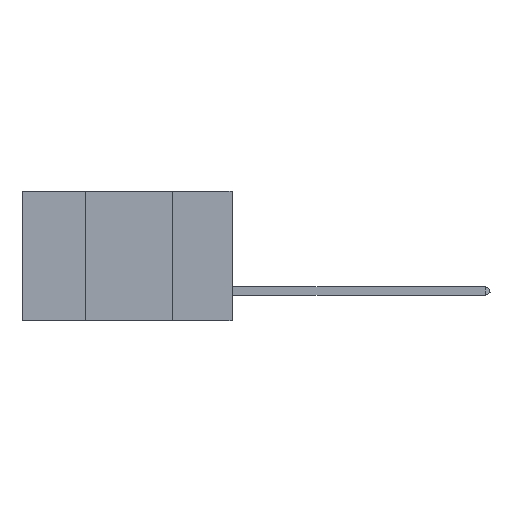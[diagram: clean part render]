
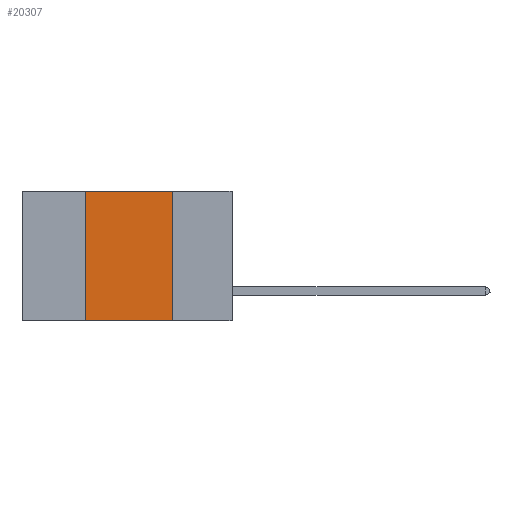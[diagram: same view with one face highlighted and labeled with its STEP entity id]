
A CAD part, left-side view. The second image highlights one B-rep face of the part: STEP entity #20307.
In plain terms, the highlighted planar face has unit normal (-1, 0, 0).
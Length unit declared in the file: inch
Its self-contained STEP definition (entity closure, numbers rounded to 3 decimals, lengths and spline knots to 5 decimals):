
#463 = DIRECTION ( 'NONE',  ( 1., 0., 0. ) ) ;
#1718 = LINE ( 'NONE', #19362, #26135 ) ;
#1923 = CARTESIAN_POINT ( 'NONE',  ( 0., 0.6, -0.37 ) ) ;
#3035 = PLANE ( 'NONE',  #10450 ) ;
#4197 = CARTESIAN_POINT ( 'NONE',  ( 0., 0.17, -0.37 ) ) ;
#4352 = EDGE_CURVE ( 'NONE', #13098, #8558, #22935, .T. ) ;
#4533 = CARTESIAN_POINT ( 'NONE',  ( 0., 0.42, 0. ) ) ;
#4908 = LINE ( 'NONE', #24232, #18678 ) ;
#5317 = DIRECTION ( 'NONE',  ( 0., 0., -1. ) ) ;
#5902 = CARTESIAN_POINT ( 'NONE',  ( 0., 0.42, -0.37 ) ) ;
#6944 = VERTEX_POINT ( 'NONE', #4197 ) ;
#8126 = LINE ( 'NONE', #1923, #8457 ) ;
#8192 = EDGE_CURVE ( 'NONE', #13098, #6944, #8126, .T. ) ;
#8457 = VECTOR ( 'NONE', #8858, 39.37008 ) ;
#8558 = VERTEX_POINT ( 'NONE', #12243 ) ;
#8695 = EDGE_CURVE ( 'NONE', #8558, #15946, #4908, .T. ) ;
#8858 = DIRECTION ( 'NONE',  ( 0., -1., 0. ) ) ;
#9001 = FACE_OUTER_BOUND ( 'NONE', #20872, .T. ) ;
#10450 = AXIS2_PLACEMENT_3D ( 'NONE', #14301, #463, #5317 ) ;
#12243 = CARTESIAN_POINT ( 'NONE',  ( 0., 0.42, 0. ) ) ;
#13098 = VERTEX_POINT ( 'NONE', #5902 ) ;
#14301 = CARTESIAN_POINT ( 'NONE',  ( 0., 0.6, 0. ) ) ;
#15802 = DIRECTION ( 'NONE',  ( 0., 0., 1. ) ) ;
#15946 = VERTEX_POINT ( 'NONE', #19304 ) ;
#16084 = ORIENTED_EDGE ( 'NONE', *, *, #4352, .F. ) ;
#18678 = VECTOR ( 'NONE', #19539, 39.37008 ) ;
#19304 = CARTESIAN_POINT ( 'NONE',  ( 0., 0.17, 0. ) ) ;
#19362 = CARTESIAN_POINT ( 'NONE',  ( 0., 0.17, 0. ) ) ;
#19539 = DIRECTION ( 'NONE',  ( 0., -1., 0. ) ) ;
#20307 = ADVANCED_FACE ( 'NONE', ( #9001 ), #3035, .F. ) ;
#20872 = EDGE_LOOP ( 'NONE', ( #21194, #29105, #16084, #26406 ) ) ;
#21194 = ORIENTED_EDGE ( 'NONE', *, *, #23361, .F. ) ;
#22935 = LINE ( 'NONE', #4533, #28597 ) ;
#23361 = EDGE_CURVE ( 'NONE', #15946, #6944, #1718, .T. ) ;
#24232 = CARTESIAN_POINT ( 'NONE',  ( 0., 0.6, 0. ) ) ;
#25726 = DIRECTION ( 'NONE',  ( 0., 0., -1. ) ) ;
#26135 = VECTOR ( 'NONE', #25726, 39.37008 ) ;
#26406 = ORIENTED_EDGE ( 'NONE', *, *, #8192, .T. ) ;
#28597 = VECTOR ( 'NONE', #15802, 39.37008 ) ;
#29105 = ORIENTED_EDGE ( 'NONE', *, *, #8695, .F. ) ;
